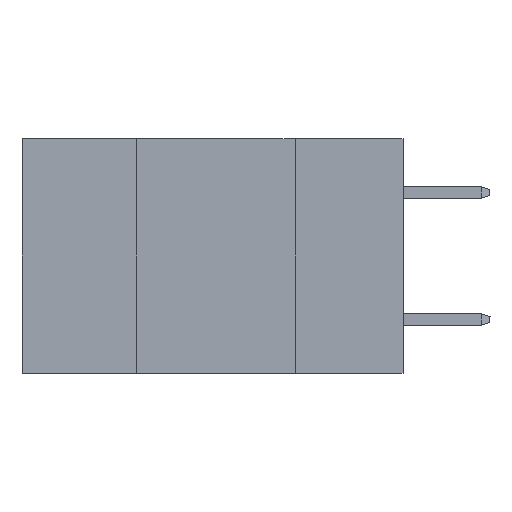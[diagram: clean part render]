
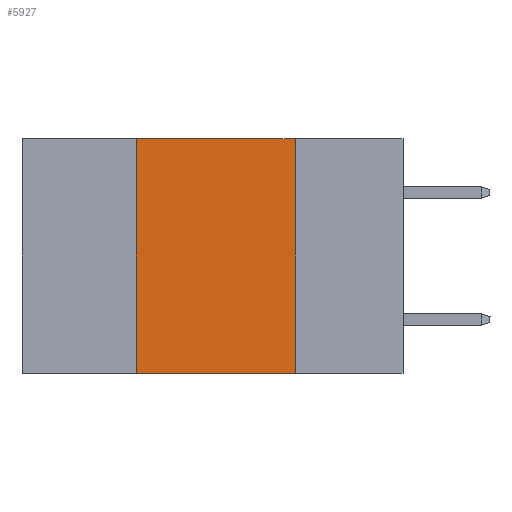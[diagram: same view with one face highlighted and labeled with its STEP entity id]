
A CAD part, left-side view. The second image highlights one B-rep face of the part: STEP entity #5927.
In plain terms, the highlighted planar face has unit normal (-1, 0, 0).
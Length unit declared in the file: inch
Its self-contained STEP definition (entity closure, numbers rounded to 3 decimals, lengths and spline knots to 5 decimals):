
#230 = EDGE_CURVE ( 'NONE', #21622, #5246, #11792, .T. ) ;
#3215 = VECTOR ( 'NONE', #7712, 39.37008 ) ;
#5246 = VERTEX_POINT ( 'NONE', #27294 ) ;
#5506 = VECTOR ( 'NONE', #14373, 39.37008 ) ;
#5555 = CARTESIAN_POINT ( 'NONE',  ( 0., 0.6, 0. ) ) ;
#5568 = CARTESIAN_POINT ( 'NONE',  ( 0., 0.17, 0. ) ) ;
#5801 = EDGE_LOOP ( 'NONE', ( #6766, #27482, #12860, #27866 ) ) ;
#5927 = ADVANCED_FACE ( 'NONE', ( #11447 ), #11003, .F. ) ;
#6650 = CARTESIAN_POINT ( 'NONE',  ( 0., 0.17, -0.37 ) ) ;
#6766 = ORIENTED_EDGE ( 'NONE', *, *, #17345, .F. ) ;
#6817 = DIRECTION ( 'NONE',  ( 1., 0., 0. ) ) ;
#7712 = DIRECTION ( 'NONE',  ( 0., -1., 0. ) ) ;
#7870 = DIRECTION ( 'NONE',  ( 0., 0., -1. ) ) ;
#8245 = CARTESIAN_POINT ( 'NONE',  ( 0., 0.42, -0.37 ) ) ;
#9674 = VERTEX_POINT ( 'NONE', #19073 ) ;
#9887 = LINE ( 'NONE', #27598, #3215 ) ;
#11003 = PLANE ( 'NONE',  #24493 ) ;
#11447 = FACE_OUTER_BOUND ( 'NONE', #5801, .T. ) ;
#11792 = LINE ( 'NONE', #20784, #14089 ) ;
#12860 = ORIENTED_EDGE ( 'NONE', *, *, #230, .F. ) ;
#13322 = CARTESIAN_POINT ( 'NONE',  ( 0., 0.6, 0. ) ) ;
#14089 = VECTOR ( 'NONE', #18576, 39.37008 ) ;
#14373 = DIRECTION ( 'NONE',  ( 0., -1., 0. ) ) ;
#17345 = EDGE_CURVE ( 'NONE', #9674, #17737, #20964, .T. ) ;
#17737 = VERTEX_POINT ( 'NONE', #6650 ) ;
#18576 = DIRECTION ( 'NONE',  ( 0., 0., 1. ) ) ;
#19073 = CARTESIAN_POINT ( 'NONE',  ( 0., 0.17, 0. ) ) ;
#19893 = EDGE_CURVE ( 'NONE', #21622, #17737, #9887, .T. ) ;
#19911 = EDGE_CURVE ( 'NONE', #5246, #9674, #25435, .T. ) ;
#20784 = CARTESIAN_POINT ( 'NONE',  ( 0., 0.42, 0. ) ) ;
#20964 = LINE ( 'NONE', #5568, #25772 ) ;
#21622 = VERTEX_POINT ( 'NONE', #8245 ) ;
#24493 = AXIS2_PLACEMENT_3D ( 'NONE', #13322, #6817, #24542 ) ;
#24542 = DIRECTION ( 'NONE',  ( 0., 0., -1. ) ) ;
#25435 = LINE ( 'NONE', #5555, #5506 ) ;
#25772 = VECTOR ( 'NONE', #7870, 39.37008 ) ;
#27294 = CARTESIAN_POINT ( 'NONE',  ( 0., 0.42, 0. ) ) ;
#27482 = ORIENTED_EDGE ( 'NONE', *, *, #19911, .F. ) ;
#27598 = CARTESIAN_POINT ( 'NONE',  ( 0., 0.6, -0.37 ) ) ;
#27866 = ORIENTED_EDGE ( 'NONE', *, *, #19893, .T. ) ;
